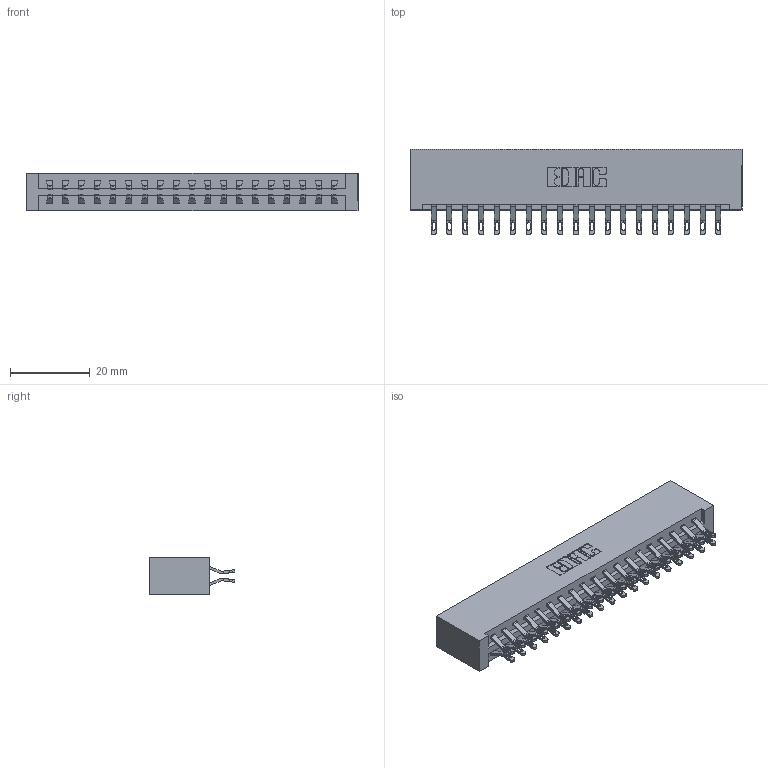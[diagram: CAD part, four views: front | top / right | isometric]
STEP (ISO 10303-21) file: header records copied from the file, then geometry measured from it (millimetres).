
FILE_DESCRIPTION (( 'STEP AP203' ), '1' );
FILE_NAME ('337-038-555-201.STEP', '2018-08-08T05:15:20', ( '' ), ( '' ), 'SwSTEP 2.0', 'SolidWorks 2016', '' );
FILE_SCHEMA (( 'CONFIG_CONTROL_DESIGN' ));
Length unit declared in the file: inch
Products named in the file (3): 345-292-001_555 Tail; 337-038-555-201; 337 Part_No Mounting Lugs
Assembly tree (39 placements, depth 2):
  337-038-555-201
    337 Part_No Mounting Lugs
    345-292-001_555 Tail  x38
Bounding box: 83.16 x 21.47 x 9.4 mm (x, y, z)
Volume: 9328.8 mm3; surface area: 10794.3 mm2
Topology: 39 solids, 39 shells, 2386 faces, 7469 edges, 4978 vertices
Faces by surface type: plane 1434, cylinder 952
Entity records: 17755 total; most frequent: CARTESIAN_POINT 3044, ORIENTED_EDGE 2950, DIRECTION 2595, EDGE_CURVE 1475, VECTOR 1335, LINE 1335, VERTEX_POINT 982, AXIS2_PLACEMENT_3D 630
